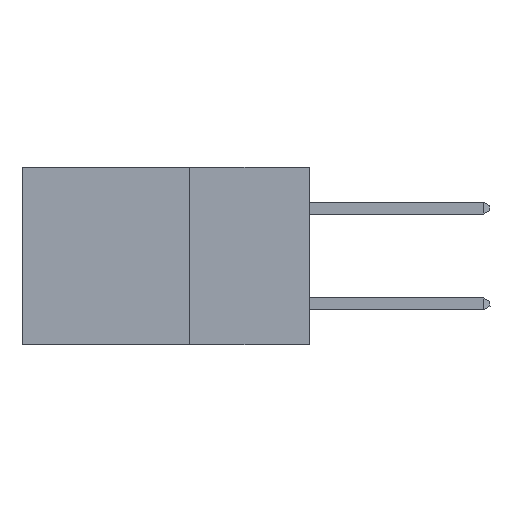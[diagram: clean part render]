
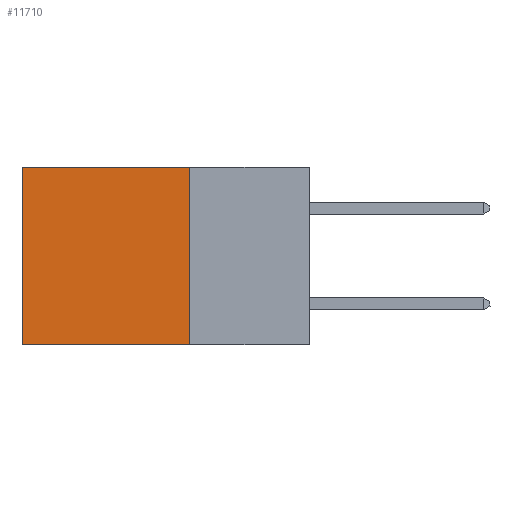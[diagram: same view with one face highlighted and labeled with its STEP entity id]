
A CAD part, left-side view. The second image highlights one B-rep face of the part: STEP entity #11710.
In plain terms, the highlighted planar face has unit normal (-1, 0, 0).
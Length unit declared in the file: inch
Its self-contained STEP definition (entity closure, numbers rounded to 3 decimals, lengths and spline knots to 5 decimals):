
#812 = VERTEX_POINT ( 'NONE', #3049 ) ;
#1383 = CARTESIAN_POINT ( 'NONE',  ( 0.2875, 0.25, 0. ) ) ;
#1954 = EDGE_CURVE ( 'NONE', #7405, #812, #8834, .T. ) ;
#2053 = LINE ( 'NONE', #16193, #15436 ) ;
#2856 = CARTESIAN_POINT ( 'NONE',  ( 0.2875, 0.25, -0.37 ) ) ;
#3049 = CARTESIAN_POINT ( 'NONE',  ( 0.2875, 0.6, 0. ) ) ;
#3219 = EDGE_LOOP ( 'NONE', ( #6426, #6378, #5851, #17054 ) ) ;
#3851 = DIRECTION ( 'NONE',  ( 0., 0., -1. ) ) ;
#4132 = CARTESIAN_POINT ( 'NONE',  ( 0.2875, 0.6, -0.37 ) ) ;
#4328 = VERTEX_POINT ( 'NONE', #2856 ) ;
#4483 = EDGE_CURVE ( 'NONE', #4328, #16384, #4661, .T. ) ;
#4661 = LINE ( 'NONE', #13985, #14766 ) ;
#5851 = ORIENTED_EDGE ( 'NONE', *, *, #8484, .F. ) ;
#6378 = ORIENTED_EDGE ( 'NONE', *, *, #4483, .F. ) ;
#6426 = ORIENTED_EDGE ( 'NONE', *, *, #12698, .T. ) ;
#6590 = LINE ( 'NONE', #7091, #10130 ) ;
#7091 = CARTESIAN_POINT ( 'NONE',  ( 0.2875, 0.6, 0. ) ) ;
#7405 = VERTEX_POINT ( 'NONE', #1383 ) ;
#8020 = PLANE ( 'NONE',  #14967 ) ;
#8484 = EDGE_CURVE ( 'NONE', #7405, #4328, #2053, .T. ) ;
#8570 = DIRECTION ( 'NONE',  ( 0., 0., -1. ) ) ;
#8834 = LINE ( 'NONE', #12122, #11910 ) ;
#10130 = VECTOR ( 'NONE', #17368, 39.37008 ) ;
#10844 = DIRECTION ( 'NONE',  ( 0., 1., 0. ) ) ;
#10988 = FACE_OUTER_BOUND ( 'NONE', #3219, .T. ) ;
#11710 = ADVANCED_FACE ( 'NONE', ( #10988 ), #8020, .F. ) ;
#11910 = VECTOR ( 'NONE', #10844, 39.37008 ) ;
#11985 = DIRECTION ( 'NONE',  ( 1., 0., 0. ) ) ;
#12122 = CARTESIAN_POINT ( 'NONE',  ( 0.2875, 0.25, 0. ) ) ;
#12698 = EDGE_CURVE ( 'NONE', #812, #16384, #6590, .T. ) ;
#13240 = DIRECTION ( 'NONE',  ( 0., 1., 0. ) ) ;
#13985 = CARTESIAN_POINT ( 'NONE',  ( 0.2875, 0.25, -0.37 ) ) ;
#14766 = VECTOR ( 'NONE', #13240, 39.37008 ) ;
#14967 = AXIS2_PLACEMENT_3D ( 'NONE', #15690, #11985, #3851 ) ;
#15436 = VECTOR ( 'NONE', #8570, 39.37008 ) ;
#15690 = CARTESIAN_POINT ( 'NONE',  ( 0.2875, 0.25, 0. ) ) ;
#16193 = CARTESIAN_POINT ( 'NONE',  ( 0.2875, 0.25, 0. ) ) ;
#16384 = VERTEX_POINT ( 'NONE', #4132 ) ;
#17054 = ORIENTED_EDGE ( 'NONE', *, *, #1954, .T. ) ;
#17368 = DIRECTION ( 'NONE',  ( 0., 0., -1. ) ) ;
